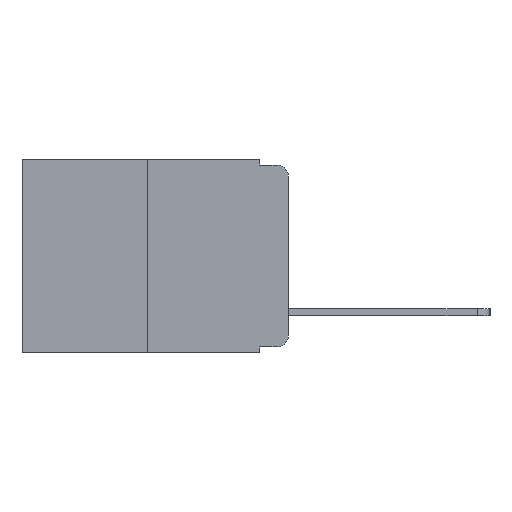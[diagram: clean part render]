
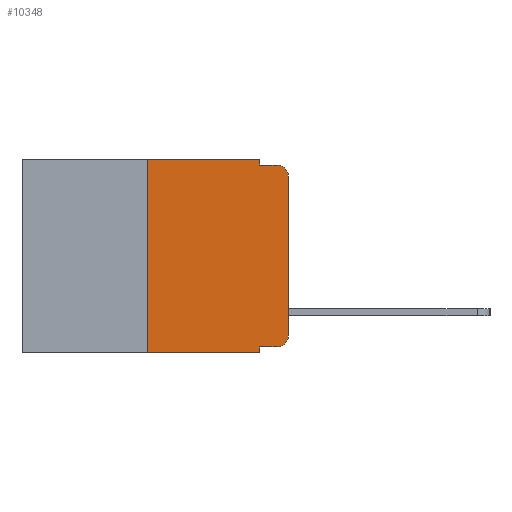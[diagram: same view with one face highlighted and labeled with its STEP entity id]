
A CAD part, left-side view. The second image highlights one B-rep face of the part: STEP entity #10348.
In plain terms, the highlighted planar face has unit normal (-1, 0, 0).
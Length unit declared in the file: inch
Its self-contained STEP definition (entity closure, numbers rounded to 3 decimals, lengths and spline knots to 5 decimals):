
#92 = ORIENTED_EDGE ( 'NONE', *, *, #12078, .F. ) ;
#169 = VERTEX_POINT ( 'NONE', #6803 ) ;
#430 = ORIENTED_EDGE ( 'NONE', *, *, #9464, .T. ) ;
#439 = VERTEX_POINT ( 'NONE', #9159 ) ;
#661 = ORIENTED_EDGE ( 'NONE', *, *, #5727, .T. ) ;
#1316 = AXIS2_PLACEMENT_3D ( 'NONE', #8021, #17397, #9431 ) ;
#1549 = DIRECTION ( 'NONE',  ( 0., 0., -1. ) ) ;
#1803 = CARTESIAN_POINT ( 'NONE',  ( 0., 0.473, -0.343 ) ) ;
#1913 = CIRCLE ( 'NONE', #1316, 0.02 ) ;
#2502 = VERTEX_POINT ( 'NONE', #12335 ) ;
#2740 = ORIENTED_EDGE ( 'NONE', *, *, #4092, .F. ) ;
#2970 = ORIENTED_EDGE ( 'NONE', *, *, #9211, .T. ) ;
#3116 = ORIENTED_EDGE ( 'NONE', *, *, #10693, .T. ) ;
#3513 = CARTESIAN_POINT ( 'NONE',  ( 0., 0.473, 0. ) ) ;
#3837 = VECTOR ( 'NONE', #10485, 39.37008 ) ;
#4083 = VERTEX_POINT ( 'NONE', #10750 ) ;
#4092 = EDGE_CURVE ( 'NONE', #12128, #2502, #11464, .T. ) ;
#4202 = EDGE_CURVE ( 'NONE', #5576, #169, #16806, .T. ) ;
#4771 = VECTOR ( 'NONE', #5003, 39.37008 ) ;
#4975 = DIRECTION ( 'NONE',  ( 0., 0., -1. ) ) ;
#5003 = DIRECTION ( 'NONE',  ( 0., -1., 0. ) ) ;
#5075 = CARTESIAN_POINT ( 'NONE',  ( 0., 0., -0.03 ) ) ;
#5140 = LINE ( 'NONE', #1803, #8113 ) ;
#5309 = EDGE_CURVE ( 'NONE', #169, #10020, #15362, .T. ) ;
#5576 = VERTEX_POINT ( 'NONE', #8978 ) ;
#5727 = EDGE_CURVE ( 'NONE', #12128, #4083, #11951, .T. ) ;
#5945 = VECTOR ( 'NONE', #12017, 39.37008 ) ;
#6420 = VERTEX_POINT ( 'NONE', #5075 ) ;
#6423 = PLANE ( 'NONE',  #17221 ) ;
#6803 = CARTESIAN_POINT ( 'NONE',  ( 0., 0.051, -0.01 ) ) ;
#6812 = ORIENTED_EDGE ( 'NONE', *, *, #16379, .T. ) ;
#6868 = ORIENTED_EDGE ( 'NONE', *, *, #4202, .F. ) ;
#6982 = LINE ( 'NONE', #7338, #17716 ) ;
#7018 = ORIENTED_EDGE ( 'NONE', *, *, #5309, .F. ) ;
#7338 = CARTESIAN_POINT ( 'NONE',  ( 0., 0., 0. ) ) ;
#8021 = CARTESIAN_POINT ( 'NONE',  ( 0., 0.02, -0.03 ) ) ;
#8113 = VECTOR ( 'NONE', #13249, 39.37008 ) ;
#8305 = CARTESIAN_POINT ( 'NONE',  ( 0., 0.02, -0.01 ) ) ;
#8791 = CIRCLE ( 'NONE', #9050, 0.02 ) ;
#8978 = CARTESIAN_POINT ( 'NONE',  ( 0., 0.051, 0. ) ) ;
#9035 = VERTEX_POINT ( 'NONE', #11259 ) ;
#9050 = AXIS2_PLACEMENT_3D ( 'NONE', #15666, #10293, #1549 ) ;
#9080 = LINE ( 'NONE', #3513, #4771 ) ;
#9159 = CARTESIAN_POINT ( 'NONE',  ( 0., 0.25, -0.343 ) ) ;
#9211 = EDGE_CURVE ( 'NONE', #4083, #9035, #8791, .T. ) ;
#9431 = DIRECTION ( 'NONE',  ( 0., 0., -1. ) ) ;
#9464 = EDGE_CURVE ( 'NONE', #439, #2502, #5140, .T. ) ;
#9520 = CARTESIAN_POINT ( 'NONE',  ( 0., 0.051, -0.333 ) ) ;
#10020 = VERTEX_POINT ( 'NONE', #8305 ) ;
#10054 = DIRECTION ( 'NONE',  ( 0., -1., 0. ) ) ;
#10293 = DIRECTION ( 'NONE',  ( -1., 0., 0. ) ) ;
#10348 = ADVANCED_FACE ( 'NONE', ( #13664 ), #6423, .F. ) ;
#10485 = DIRECTION ( 'NONE',  ( 0., 0., -1. ) ) ;
#10665 = CARTESIAN_POINT ( 'NONE',  ( 0., 0.473, 0. ) ) ;
#10693 = EDGE_CURVE ( 'NONE', #9035, #6420, #6982, .T. ) ;
#10750 = CARTESIAN_POINT ( 'NONE',  ( 0., 0.02, -0.333 ) ) ;
#10803 = VECTOR ( 'NONE', #14765, 39.37008 ) ;
#11259 = CARTESIAN_POINT ( 'NONE',  ( 0., 0., -0.313 ) ) ;
#11464 = LINE ( 'NONE', #11825, #3837 ) ;
#11536 = VECTOR ( 'NONE', #10054, 39.37008 ) ;
#11825 = CARTESIAN_POINT ( 'NONE',  ( 0., 0.051, 0. ) ) ;
#11834 = VECTOR ( 'NONE', #15663, 39.37008 ) ;
#11951 = LINE ( 'NONE', #16227, #11536 ) ;
#12017 = DIRECTION ( 'NONE',  ( 0., 0., -1. ) ) ;
#12078 = EDGE_CURVE ( 'NONE', #439, #17692, #14399, .T. ) ;
#12128 = VERTEX_POINT ( 'NONE', #9520 ) ;
#12161 = ORIENTED_EDGE ( 'NONE', *, *, #15168, .F. ) ;
#12335 = CARTESIAN_POINT ( 'NONE',  ( 0., 0.051, -0.343 ) ) ;
#13249 = DIRECTION ( 'NONE',  ( 0., -1., 0. ) ) ;
#13390 = DIRECTION ( 'NONE',  ( 1., 0., 0. ) ) ;
#13664 = FACE_OUTER_BOUND ( 'NONE', #15125, .T. ) ;
#14399 = LINE ( 'NONE', #14820, #10803 ) ;
#14765 = DIRECTION ( 'NONE',  ( 0., 0., 1. ) ) ;
#14820 = CARTESIAN_POINT ( 'NONE',  ( 0., 0.25, 0. ) ) ;
#15125 = EDGE_LOOP ( 'NONE', ( #3116, #6812, #7018, #6868, #12161, #92, #430, #2740, #661, #2970 ) ) ;
#15168 = EDGE_CURVE ( 'NONE', #17692, #5576, #9080, .T. ) ;
#15194 = CARTESIAN_POINT ( 'NONE',  ( 0., 0.25, 0. ) ) ;
#15362 = LINE ( 'NONE', #15555, #11834 ) ;
#15555 = CARTESIAN_POINT ( 'NONE',  ( 0., 0.051, -0.01 ) ) ;
#15663 = DIRECTION ( 'NONE',  ( 0., -1., 0. ) ) ;
#15666 = CARTESIAN_POINT ( 'NONE',  ( 0., 0.02, -0.313 ) ) ;
#16227 = CARTESIAN_POINT ( 'NONE',  ( 0., 0.051, -0.333 ) ) ;
#16379 = EDGE_CURVE ( 'NONE', #6420, #10020, #1913, .T. ) ;
#16791 = DIRECTION ( 'NONE',  ( 0., 0., 1. ) ) ;
#16806 = LINE ( 'NONE', #17396, #5945 ) ;
#17221 = AXIS2_PLACEMENT_3D ( 'NONE', #10665, #13390, #4975 ) ;
#17396 = CARTESIAN_POINT ( 'NONE',  ( 0., 0.051, 0. ) ) ;
#17397 = DIRECTION ( 'NONE',  ( -1., 0., 0. ) ) ;
#17692 = VERTEX_POINT ( 'NONE', #15194 ) ;
#17716 = VECTOR ( 'NONE', #16791, 39.37008 ) ;
